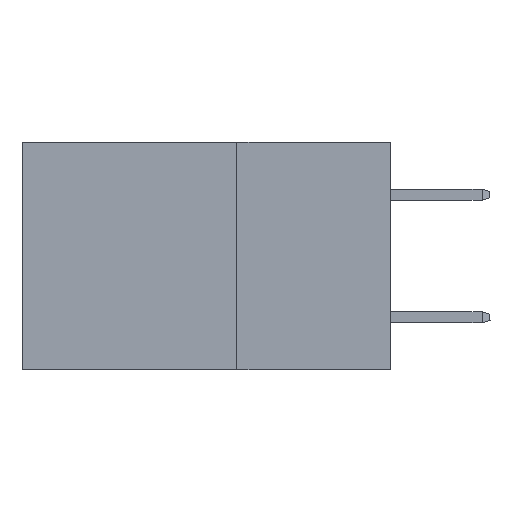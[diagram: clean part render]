
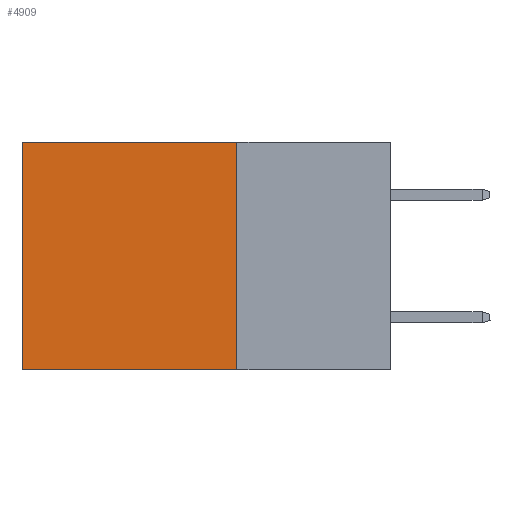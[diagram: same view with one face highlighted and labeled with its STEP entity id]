
A CAD part, left-side view. The second image highlights one B-rep face of the part: STEP entity #4909.
In plain terms, the highlighted planar face has unit normal (-1, 0, 0).
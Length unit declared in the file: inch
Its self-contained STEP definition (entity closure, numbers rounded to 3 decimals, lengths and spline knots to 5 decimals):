
#2434 = ORIENTED_EDGE ( 'NONE', *, *, #37869, .F. ) ;
#2847 = CARTESIAN_POINT ( 'NONE',  ( 0.2875, 0.6, 0. ) ) ;
#4909 = ADVANCED_FACE ( 'NONE', ( #10803 ), #24338, .F. ) ;
#5314 = VECTOR ( 'NONE', #13493, 39.37008 ) ;
#5839 = VECTOR ( 'NONE', #26861, 39.37008 ) ;
#8011 = EDGE_CURVE ( 'NONE', #30334, #43470, #26827, .T. ) ;
#10803 = FACE_OUTER_BOUND ( 'NONE', #30545, .T. ) ;
#11672 = DIRECTION ( 'NONE',  ( 0., 0., -1. ) ) ;
#12764 = AXIS2_PLACEMENT_3D ( 'NONE', #37903, #14788, #11672 ) ;
#13493 = DIRECTION ( 'NONE',  ( 0., 0., -1. ) ) ;
#14788 = DIRECTION ( 'NONE',  ( 1., 0., 0. ) ) ;
#15375 = DIRECTION ( 'NONE',  ( 0., 1., 0. ) ) ;
#18436 = LINE ( 'NONE', #34054, #31463 ) ;
#19294 = EDGE_CURVE ( 'NONE', #25424, #30334, #28918, .T. ) ;
#20685 = ORIENTED_EDGE ( 'NONE', *, *, #8011, .T. ) ;
#22064 = CARTESIAN_POINT ( 'NONE',  ( 0.2875, 0.6, 0. ) ) ;
#23531 = CARTESIAN_POINT ( 'NONE',  ( 0.2875, 0.25, -0.37 ) ) ;
#23719 = ORIENTED_EDGE ( 'NONE', *, *, #19294, .T. ) ;
#23800 = CARTESIAN_POINT ( 'NONE',  ( 0.2875, 0.25, 0. ) ) ;
#24338 = PLANE ( 'NONE',  #12764 ) ;
#25424 = VERTEX_POINT ( 'NONE', #23800 ) ;
#25559 = VERTEX_POINT ( 'NONE', #36956 ) ;
#26827 = LINE ( 'NONE', #2847, #5314 ) ;
#26861 = DIRECTION ( 'NONE',  ( 0., 1., 0. ) ) ;
#28918 = LINE ( 'NONE', #39159, #43066 ) ;
#30334 = VERTEX_POINT ( 'NONE', #22064 ) ;
#30538 = ORIENTED_EDGE ( 'NONE', *, *, #36225, .F. ) ;
#30545 = EDGE_LOOP ( 'NONE', ( #20685, #30538, #2434, #23719 ) ) ;
#31463 = VECTOR ( 'NONE', #40931, 39.37008 ) ;
#33307 = LINE ( 'NONE', #23531, #5839 ) ;
#34002 = CARTESIAN_POINT ( 'NONE',  ( 0.2875, 0.6, -0.37 ) ) ;
#34054 = CARTESIAN_POINT ( 'NONE',  ( 0.2875, 0.25, 0. ) ) ;
#36225 = EDGE_CURVE ( 'NONE', #25559, #43470, #33307, .T. ) ;
#36956 = CARTESIAN_POINT ( 'NONE',  ( 0.2875, 0.25, -0.37 ) ) ;
#37869 = EDGE_CURVE ( 'NONE', #25424, #25559, #18436, .T. ) ;
#37903 = CARTESIAN_POINT ( 'NONE',  ( 0.2875, 0.25, 0. ) ) ;
#39159 = CARTESIAN_POINT ( 'NONE',  ( 0.2875, 0.25, 0. ) ) ;
#40931 = DIRECTION ( 'NONE',  ( 0., 0., -1. ) ) ;
#43066 = VECTOR ( 'NONE', #15375, 39.37008 ) ;
#43470 = VERTEX_POINT ( 'NONE', #34002 ) ;
